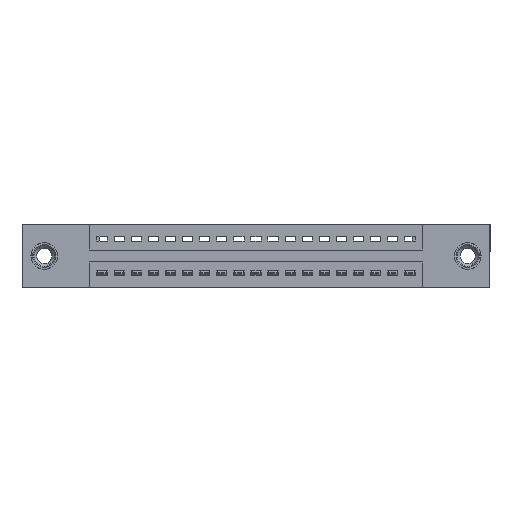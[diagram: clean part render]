
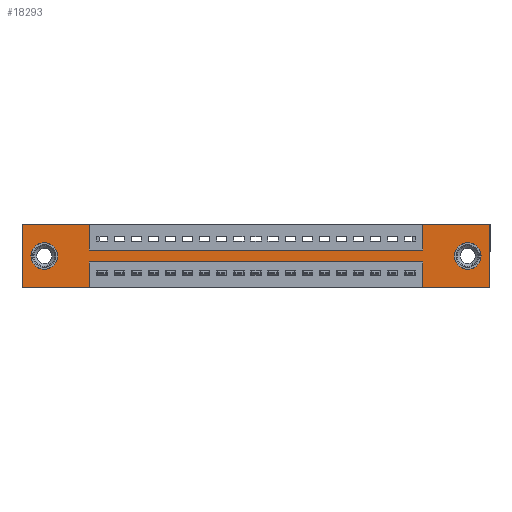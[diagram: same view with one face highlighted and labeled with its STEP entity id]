
A CAD part, front view. The second image highlights one B-rep face of the part: STEP entity #18293.
In plain terms, the highlighted planar face has unit normal (0, -1, 0).
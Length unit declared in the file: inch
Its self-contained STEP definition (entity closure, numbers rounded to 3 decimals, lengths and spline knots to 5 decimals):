
#278 = ORIENTED_EDGE ( 'NONE', *, *, #19145, .F. ) ;
#383 = CARTESIAN_POINT ( 'NONE',  ( 0.3925, 0., 0. ) ) ;
#437 = CARTESIAN_POINT ( 'NONE',  ( 0.3925, 0., -0.37 ) ) ;
#492 = DIRECTION ( 'NONE',  ( 1., 0., 0. ) ) ;
#1008 = CARTESIAN_POINT ( 'NONE',  ( 0.3925, 0., -0.15 ) ) ;
#1476 = CARTESIAN_POINT ( 'NONE',  ( 0.3925, 0., -0.22 ) ) ;
#1505 = VECTOR ( 'NONE', #492, 39.37008 ) ;
#1573 = DIRECTION ( 'NONE',  ( 1., 0., 0. ) ) ;
#2009 = DIRECTION ( 'NONE',  ( 0., 0., -1. ) ) ;
#2107 = FACE_OUTER_BOUND ( 'NONE', #11419, .T. ) ;
#2143 = DIRECTION ( 'NONE',  ( 0., 0., -1. ) ) ;
#2276 = VECTOR ( 'NONE', #4564, 39.37008 ) ;
#2306 = VERTEX_POINT ( 'NONE', #14600 ) ;
#2337 = CARTESIAN_POINT ( 'NONE',  ( 0., 0., -0.37 ) ) ;
#2578 = DIRECTION ( 'NONE',  ( 0., 0., 1. ) ) ;
#2589 = EDGE_CURVE ( 'NONE', #19282, #2607, #12148, .T. ) ;
#2607 = VERTEX_POINT ( 'NONE', #8177 ) ;
#3029 = CARTESIAN_POINT ( 'NONE',  ( 0., 0., 0. ) ) ;
#3170 = CARTESIAN_POINT ( 'NONE',  ( 0., 0., -0.37 ) ) ;
#3580 = CIRCLE ( 'NONE', #16169, 0.078 ) ;
#3601 = DIRECTION ( 'NONE',  ( 0., 1., 0. ) ) ;
#3667 = VERTEX_POINT ( 'NONE', #10968 ) ;
#3766 = VERTEX_POINT ( 'NONE', #10785 ) ;
#3968 = AXIS2_PLACEMENT_3D ( 'NONE', #11319, #3601, #8221 ) ;
#4364 = CARTESIAN_POINT ( 'NONE',  ( 0., 0., 0. ) ) ;
#4450 = VECTOR ( 'NONE', #14396, 39.37008 ) ;
#4564 = DIRECTION ( 'NONE',  ( -1., 0., 0. ) ) ;
#5015 = PLANE ( 'NONE',  #5614 ) ;
#5126 = DIRECTION ( 'NONE',  ( 0., 0., 1. ) ) ;
#5272 = LINE ( 'NONE', #383, #6899 ) ;
#5287 = DIRECTION ( 'NONE',  ( -1., 0., 0. ) ) ;
#5379 = CIRCLE ( 'NONE', #9385, 0.078 ) ;
#5593 = CARTESIAN_POINT ( 'NONE',  ( 0.3925, 0., -0.37 ) ) ;
#5598 = ORIENTED_EDGE ( 'NONE', *, *, #9516, .T. ) ;
#5614 = AXIS2_PLACEMENT_3D ( 'NONE', #15454, #6656, #8145 ) ;
#6529 = DIRECTION ( 'NONE',  ( 0., 0., -1. ) ) ;
#6584 = EDGE_CURVE ( 'NONE', #14298, #9182, #8494, .T. ) ;
#6656 = DIRECTION ( 'NONE',  ( 0., -1., 0. ) ) ;
#6879 = ORIENTED_EDGE ( 'NONE', *, *, #8277, .F. ) ;
#6883 = ORIENTED_EDGE ( 'NONE', *, *, #16016, .F. ) ;
#6899 = VECTOR ( 'NONE', #2009, 39.37008 ) ;
#6914 = CIRCLE ( 'NONE', #3968, 0.078 ) ;
#7291 = VECTOR ( 'NONE', #14775, 39.37008 ) ;
#7423 = EDGE_CURVE ( 'NONE', #3766, #19224, #14050, .T. ) ;
#7664 = LINE ( 'NONE', #1476, #2276 ) ;
#7964 = EDGE_CURVE ( 'NONE', #19224, #16495, #10314, .T. ) ;
#8092 = DIRECTION ( 'NONE',  ( 0., 1., 0. ) ) ;
#8145 = DIRECTION ( 'NONE',  ( 0., 0., -1. ) ) ;
#8177 = CARTESIAN_POINT ( 'NONE',  ( 2.735, 0., 0. ) ) ;
#8221 = DIRECTION ( 'NONE',  ( 0., 0., 1. ) ) ;
#8277 = EDGE_CURVE ( 'NONE', #16495, #18424, #19226, .T. ) ;
#8364 = CARTESIAN_POINT ( 'NONE',  ( 0., 0., 0. ) ) ;
#8494 = LINE ( 'NONE', #11030, #10348 ) ;
#8612 = CARTESIAN_POINT ( 'NONE',  ( 2.3425, 0., -0.22 ) ) ;
#9067 = ORIENTED_EDGE ( 'NONE', *, *, #10224, .F. ) ;
#9074 = VERTEX_POINT ( 'NONE', #14418 ) ;
#9142 = VECTOR ( 'NONE', #6529, 39.37008 ) ;
#9182 = VERTEX_POINT ( 'NONE', #8612 ) ;
#9307 = CARTESIAN_POINT ( 'NONE',  ( 0., 0., -0.37 ) ) ;
#9385 = AXIS2_PLACEMENT_3D ( 'NONE', #9693, #8092, #2143 ) ;
#9490 = CARTESIAN_POINT ( 'NONE',  ( 2.3425, 0., -0.15 ) ) ;
#9516 = EDGE_CURVE ( 'NONE', #2306, #3667, #5379, .T. ) ;
#9656 = ORIENTED_EDGE ( 'NONE', *, *, #7423, .F. ) ;
#9693 = CARTESIAN_POINT ( 'NONE',  ( 2.605, 0., -0.185 ) ) ;
#10224 = EDGE_CURVE ( 'NONE', #9182, #3766, #7664, .T. ) ;
#10314 = LINE ( 'NONE', #9307, #15927 ) ;
#10348 = VECTOR ( 'NONE', #5126, 39.37008 ) ;
#10426 = EDGE_CURVE ( 'NONE', #17154, #19282, #16773, .T. ) ;
#10610 = LINE ( 'NONE', #18555, #1505 ) ;
#10612 = ORIENTED_EDGE ( 'NONE', *, *, #6584, .F. ) ;
#10785 = CARTESIAN_POINT ( 'NONE',  ( 0.3925, 0., -0.22 ) ) ;
#10935 = LINE ( 'NONE', #11099, #16556 ) ;
#10968 = CARTESIAN_POINT ( 'NONE',  ( 2.605, 0., -0.107 ) ) ;
#11030 = CARTESIAN_POINT ( 'NONE',  ( 2.3425, 0., -0.37 ) ) ;
#11099 = CARTESIAN_POINT ( 'NONE',  ( 2.735, 0., 0. ) ) ;
#11207 = FACE_BOUND ( 'NONE', #16918, .T. ) ;
#11300 = DIRECTION ( 'NONE',  ( 0., 1., 0. ) ) ;
#11319 = CARTESIAN_POINT ( 'NONE',  ( 0.13, 0., -0.185 ) ) ;
#11419 = EDGE_LOOP ( 'NONE', ( #9656, #9067, #10612, #17676, #278, #13592, #15390, #11502, #6883, #18817, #6879, #14007 ) ) ;
#11502 = ORIENTED_EDGE ( 'NONE', *, *, #18584, .F. ) ;
#11883 = EDGE_CURVE ( 'NONE', #18424, #17109, #10610, .T. ) ;
#11894 = EDGE_CURVE ( 'NONE', #19064, #9074, #15528, .T. ) ;
#12060 = LINE ( 'NONE', #2337, #15100 ) ;
#12148 = LINE ( 'NONE', #3029, #18019 ) ;
#12326 = CARTESIAN_POINT ( 'NONE',  ( 0.3925, 0., 0. ) ) ;
#12578 = CARTESIAN_POINT ( 'NONE',  ( 0.13, 0., -0.185 ) ) ;
#12790 = DIRECTION ( 'NONE',  ( -1., 0., 0. ) ) ;
#12796 = VECTOR ( 'NONE', #16908, 39.37008 ) ;
#12973 = ORIENTED_EDGE ( 'NONE', *, *, #13819, .T. ) ;
#12998 = CARTESIAN_POINT ( 'NONE',  ( 2.3425, 0., 0. ) ) ;
#13592 = ORIENTED_EDGE ( 'NONE', *, *, #2589, .F. ) ;
#13721 = DIRECTION ( 'NONE',  ( 0., 1., 0. ) ) ;
#13790 = FACE_BOUND ( 'NONE', #16043, .T. ) ;
#13819 = EDGE_CURVE ( 'NONE', #3667, #2306, #3580, .T. ) ;
#13849 = DIRECTION ( 'NONE',  ( 0., 0., -1. ) ) ;
#13982 = CARTESIAN_POINT ( 'NONE',  ( 0.13, 0., -0.263 ) ) ;
#14007 = ORIENTED_EDGE ( 'NONE', *, *, #7964, .F. ) ;
#14050 = LINE ( 'NONE', #437, #9142 ) ;
#14089 = EDGE_CURVE ( 'NONE', #16236, #14298, #12060, .T. ) ;
#14239 = DIRECTION ( 'NONE',  ( 0., 0., -1. ) ) ;
#14298 = VERTEX_POINT ( 'NONE', #17323 ) ;
#14326 = CARTESIAN_POINT ( 'NONE',  ( 2.735, 0., -0.37 ) ) ;
#14396 = DIRECTION ( 'NONE',  ( 1., 0., 0. ) ) ;
#14406 = ORIENTED_EDGE ( 'NONE', *, *, #15576, .T. ) ;
#14418 = CARTESIAN_POINT ( 'NONE',  ( 0.13, 0., -0.107 ) ) ;
#14600 = CARTESIAN_POINT ( 'NONE',  ( 2.605, 0., -0.263 ) ) ;
#14775 = DIRECTION ( 'NONE',  ( 0., 0., 1. ) ) ;
#15100 = VECTOR ( 'NONE', #12790, 39.37008 ) ;
#15390 = ORIENTED_EDGE ( 'NONE', *, *, #10426, .F. ) ;
#15454 = CARTESIAN_POINT ( 'NONE',  ( 0., 0., -0.37 ) ) ;
#15528 = CIRCLE ( 'NONE', #16275, 0.078 ) ;
#15576 = EDGE_CURVE ( 'NONE', #9074, #19064, #6914, .T. ) ;
#15653 = LINE ( 'NONE', #1008, #4450 ) ;
#15927 = VECTOR ( 'NONE', #5287, 39.37008 ) ;
#16016 = EDGE_CURVE ( 'NONE', #17109, #17361, #5272, .T. ) ;
#16043 = EDGE_LOOP ( 'NONE', ( #14406, #18995 ) ) ;
#16169 = AXIS2_PLACEMENT_3D ( 'NONE', #16811, #13721, #13849 ) ;
#16236 = VERTEX_POINT ( 'NONE', #14326 ) ;
#16275 = AXIS2_PLACEMENT_3D ( 'NONE', #12578, #11300, #2578 ) ;
#16495 = VERTEX_POINT ( 'NONE', #3170 ) ;
#16556 = VECTOR ( 'NONE', #14239, 39.37008 ) ;
#16773 = LINE ( 'NONE', #18507, #12796 ) ;
#16811 = CARTESIAN_POINT ( 'NONE',  ( 2.605, 0., -0.185 ) ) ;
#16908 = DIRECTION ( 'NONE',  ( 0., 0., 1. ) ) ;
#16918 = EDGE_LOOP ( 'NONE', ( #12973, #5598 ) ) ;
#17109 = VERTEX_POINT ( 'NONE', #12326 ) ;
#17154 = VERTEX_POINT ( 'NONE', #9490 ) ;
#17323 = CARTESIAN_POINT ( 'NONE',  ( 2.3425, 0., -0.37 ) ) ;
#17361 = VERTEX_POINT ( 'NONE', #19090 ) ;
#17676 = ORIENTED_EDGE ( 'NONE', *, *, #14089, .F. ) ;
#18019 = VECTOR ( 'NONE', #1573, 39.37008 ) ;
#18293 = ADVANCED_FACE ( 'NONE', ( #11207, #13790, #2107 ), #5015, .T. ) ;
#18424 = VERTEX_POINT ( 'NONE', #8364 ) ;
#18507 = CARTESIAN_POINT ( 'NONE',  ( 2.3425, 0., 0. ) ) ;
#18555 = CARTESIAN_POINT ( 'NONE',  ( 0., 0., 0. ) ) ;
#18584 = EDGE_CURVE ( 'NONE', #17361, #17154, #15653, .T. ) ;
#18817 = ORIENTED_EDGE ( 'NONE', *, *, #11883, .F. ) ;
#18995 = ORIENTED_EDGE ( 'NONE', *, *, #11894, .T. ) ;
#19064 = VERTEX_POINT ( 'NONE', #13982 ) ;
#19090 = CARTESIAN_POINT ( 'NONE',  ( 0.3925, 0., -0.15 ) ) ;
#19145 = EDGE_CURVE ( 'NONE', #2607, #16236, #10935, .T. ) ;
#19224 = VERTEX_POINT ( 'NONE', #5593 ) ;
#19226 = LINE ( 'NONE', #4364, #7291 ) ;
#19282 = VERTEX_POINT ( 'NONE', #12998 ) ;
